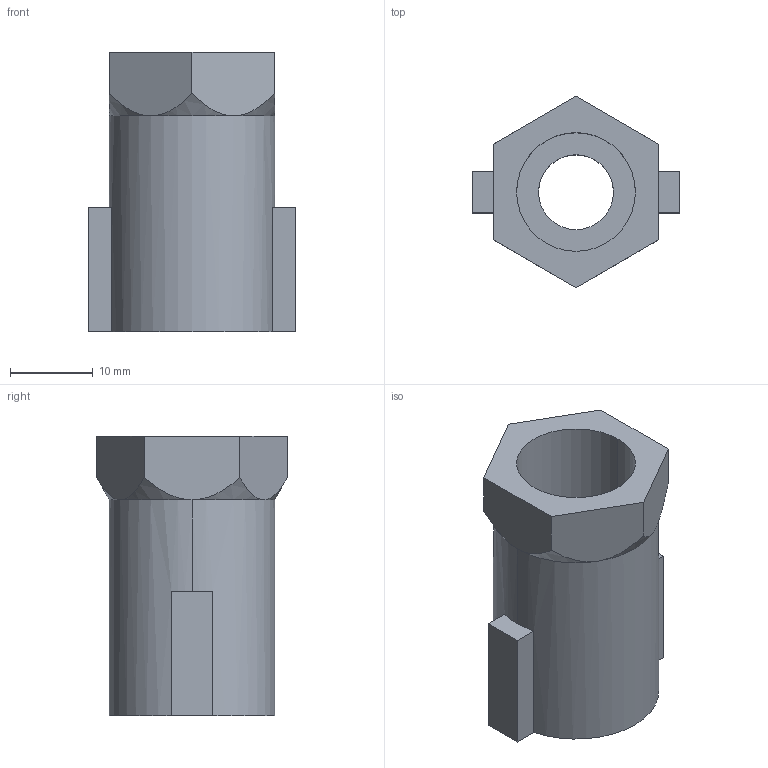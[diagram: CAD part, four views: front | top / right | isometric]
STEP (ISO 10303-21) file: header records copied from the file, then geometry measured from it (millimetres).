
FILE_DESCRIPTION (( 'STEP AP214' ), '1' );
FILE_NAME ('BarrelAndChamber.STEP', '2013-09-01T22:39:05', ( 'Asher' ), ( '' ), 'SwSTEP 2.0', 'SolidWorks 2013', '' );
FILE_SCHEMA (( 'AUTOMOTIVE_DESIGN' ));
Length unit declared in the file: millimetre
Products named in the file (1): BarrelAndChamber
Bounding box: 25 x 23.09 x 33.75 mm (x, y, z)
Volume: 7315.2 mm3; surface area: 4177.5 mm2
Topology: 1 solids, 1 shells, 35 faces, 88 edges, 56 vertices
Faces by surface type: plane 23, cylinder 6, cone 6
Entity records: 1190 total; most frequent: CARTESIAN_POINT 312, ORIENTED_EDGE 176, DIRECTION 174, EDGE_CURVE 88, AXIS2_PLACEMENT_3D 62, VERTEX_POINT 56, VECTOR 50, LINE 50
